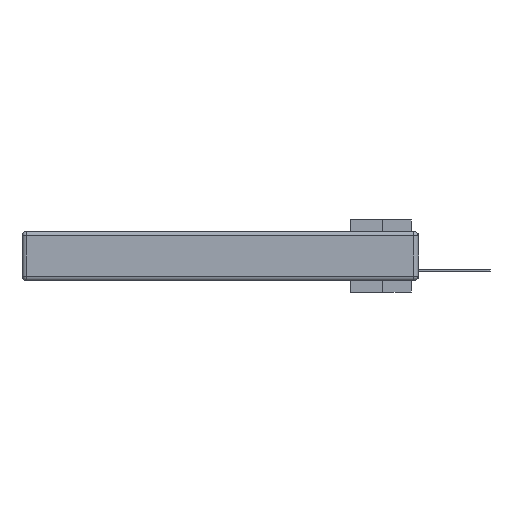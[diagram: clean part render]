
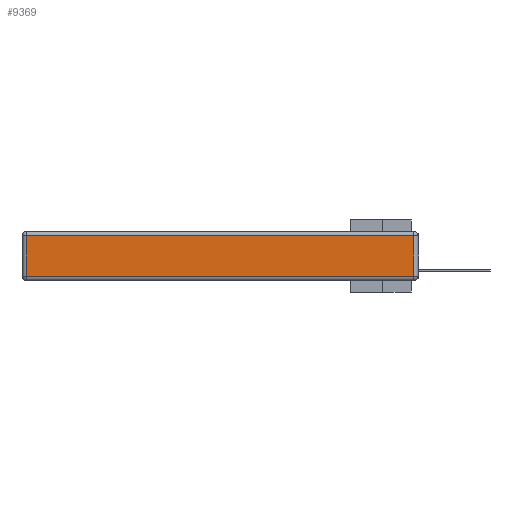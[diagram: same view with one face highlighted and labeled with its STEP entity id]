
A CAD part, left-side view. The second image highlights one B-rep face of the part: STEP entity #9369.
In plain terms, the highlighted planar face has unit normal (-1, 0, 0).
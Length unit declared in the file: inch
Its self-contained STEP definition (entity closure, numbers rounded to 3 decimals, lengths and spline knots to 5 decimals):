
#201 = CARTESIAN_POINT ( 'NONE',  ( 0., 0.03, -0.313 ) ) ;
#445 = DIRECTION ( 'NONE',  ( 0., 1., 0. ) ) ;
#2528 = EDGE_CURVE ( 'NONE', #3966, #21544, #25750, .T. ) ;
#2767 = VECTOR ( 'NONE', #445, 39.37008 ) ;
#3847 = DIRECTION ( 'NONE',  ( 0., 0., -1. ) ) ;
#3966 = VERTEX_POINT ( 'NONE', #6256 ) ;
#4112 = ORIENTED_EDGE ( 'NONE', *, *, #5510, .T. ) ;
#4996 = ORIENTED_EDGE ( 'NONE', *, *, #2528, .T. ) ;
#5510 = EDGE_CURVE ( 'NONE', #6452, #3966, #11613, .T. ) ;
#6256 = CARTESIAN_POINT ( 'NONE',  ( 0., 0.03, -0.03 ) ) ;
#6452 = VERTEX_POINT ( 'NONE', #201 ) ;
#7539 = VERTEX_POINT ( 'NONE', #9684 ) ;
#7972 = EDGE_CURVE ( 'NONE', #21544, #7539, #24302, .T. ) ;
#9369 = ADVANCED_FACE ( 'NONE', ( #12858 ), #30809, .T. ) ;
#9684 = CARTESIAN_POINT ( 'NONE',  ( 0., 2.72, -0.313 ) ) ;
#9757 = DIRECTION ( 'NONE',  ( 0., 0., 1. ) ) ;
#11613 = LINE ( 'NONE', #14283, #32285 ) ;
#12858 = FACE_OUTER_BOUND ( 'NONE', #14109, .T. ) ;
#13174 = CARTESIAN_POINT ( 'NONE',  ( 0., 0., -0.343 ) ) ;
#14109 = EDGE_LOOP ( 'NONE', ( #32312, #4112, #4996, #30522 ) ) ;
#14283 = CARTESIAN_POINT ( 'NONE',  ( 0., 0.03, -0.343 ) ) ;
#16030 = AXIS2_PLACEMENT_3D ( 'NONE', #13174, #23651, #22995 ) ;
#19151 = DIRECTION ( 'NONE',  ( 0., -1., 0. ) ) ;
#20924 = CARTESIAN_POINT ( 'NONE',  ( 0., 2.75, -0.03 ) ) ;
#21544 = VERTEX_POINT ( 'NONE', #27894 ) ;
#22132 = CARTESIAN_POINT ( 'NONE',  ( 0., 0., -0.313 ) ) ;
#22995 = DIRECTION ( 'NONE',  ( 0., 0., 1. ) ) ;
#23651 = DIRECTION ( 'NONE',  ( -1., 0., 0. ) ) ;
#24302 = LINE ( 'NONE', #24468, #30201 ) ;
#24468 = CARTESIAN_POINT ( 'NONE',  ( 0., 2.72, -0.343 ) ) ;
#25750 = LINE ( 'NONE', #20924, #2767 ) ;
#26394 = EDGE_CURVE ( 'NONE', #7539, #6452, #26805, .T. ) ;
#26574 = VECTOR ( 'NONE', #19151, 39.37008 ) ;
#26805 = LINE ( 'NONE', #22132, #26574 ) ;
#27894 = CARTESIAN_POINT ( 'NONE',  ( 0., 2.72, -0.03 ) ) ;
#30201 = VECTOR ( 'NONE', #3847, 39.37008 ) ;
#30522 = ORIENTED_EDGE ( 'NONE', *, *, #7972, .T. ) ;
#30809 = PLANE ( 'NONE',  #16030 ) ;
#32285 = VECTOR ( 'NONE', #9757, 39.37008 ) ;
#32312 = ORIENTED_EDGE ( 'NONE', *, *, #26394, .T. ) ;
